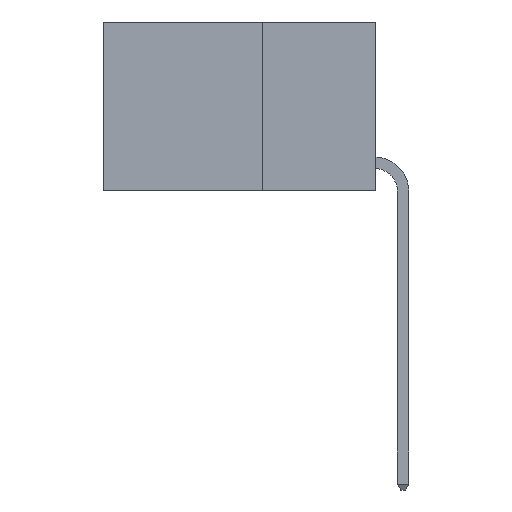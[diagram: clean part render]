
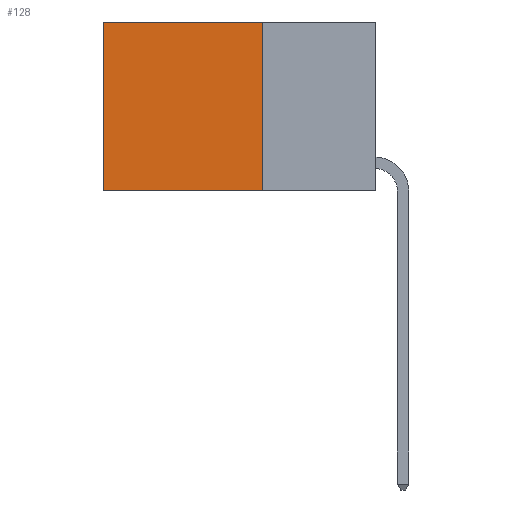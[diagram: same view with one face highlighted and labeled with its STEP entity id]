
A CAD part, left-side view. The second image highlights one B-rep face of the part: STEP entity #128.
In plain terms, the highlighted planar face has unit normal (-1, 0, 0).
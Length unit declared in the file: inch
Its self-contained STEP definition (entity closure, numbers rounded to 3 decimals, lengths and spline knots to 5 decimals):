
#128 = ADVANCED_FACE ( 'NONE', ( #4496 ), #8758, .F. ) ;
#533 = VECTOR ( 'NONE', #5621, 39.37008 ) ;
#545 = LINE ( 'NONE', #5864, #533 ) ;
#628 = EDGE_CURVE ( 'NONE', #7400, #764, #545, .T. ) ;
#734 = EDGE_LOOP ( 'NONE', ( #4826, #4939, #4992, #5083 ) ) ;
#764 = VERTEX_POINT ( 'NONE', #3080 ) ;
#966 = CARTESIAN_POINT ( 'NONE',  ( 0.2625, 0.25, 0. ) ) ;
#2362 = AXIS2_PLACEMENT_3D ( 'NONE', #4500, #7505, #8538 ) ;
#2675 = EDGE_CURVE ( 'NONE', #7400, #4387, #6437, .T. ) ;
#3080 = CARTESIAN_POINT ( 'NONE',  ( 0.2625, 0.25, -0.37 ) ) ;
#3181 = DIRECTION ( 'NONE',  ( 0., 1., 0. ) ) ;
#3272 = CARTESIAN_POINT ( 'NONE',  ( 0.2625, 0.25, 0. ) ) ;
#3732 = CARTESIAN_POINT ( 'NONE',  ( 0.2625, 0.6, -0.37 ) ) ;
#4236 = EDGE_CURVE ( 'NONE', #764, #8080, #7479, .T. ) ;
#4387 = VERTEX_POINT ( 'NONE', #5658 ) ;
#4496 = FACE_OUTER_BOUND ( 'NONE', #734, .T. ) ;
#4500 = CARTESIAN_POINT ( 'NONE',  ( 0.2625, 0.25, 0. ) ) ;
#4826 = ORIENTED_EDGE ( 'NONE', *, *, #4928, .T. ) ;
#4928 = EDGE_CURVE ( 'NONE', #4387, #8080, #5277, .T. ) ;
#4939 = ORIENTED_EDGE ( 'NONE', *, *, #4236, .F. ) ;
#4992 = ORIENTED_EDGE ( 'NONE', *, *, #628, .F. ) ;
#5083 = ORIENTED_EDGE ( 'NONE', *, *, #2675, .T. ) ;
#5277 = LINE ( 'NONE', #9057, #5325 ) ;
#5325 = VECTOR ( 'NONE', #9067, 39.37008 ) ;
#5621 = DIRECTION ( 'NONE',  ( 0., 0., -1. ) ) ;
#5658 = CARTESIAN_POINT ( 'NONE',  ( 0.2625, 0.6, 0. ) ) ;
#5864 = CARTESIAN_POINT ( 'NONE',  ( 0.2625, 0.25, 0. ) ) ;
#6437 = LINE ( 'NONE', #3272, #8177 ) ;
#7211 = VECTOR ( 'NONE', #8642, 39.37008 ) ;
#7400 = VERTEX_POINT ( 'NONE', #966 ) ;
#7479 = LINE ( 'NONE', #8477, #7211 ) ;
#7505 = DIRECTION ( 'NONE',  ( 1., 0., 0. ) ) ;
#8080 = VERTEX_POINT ( 'NONE', #3732 ) ;
#8177 = VECTOR ( 'NONE', #3181, 39.37008 ) ;
#8477 = CARTESIAN_POINT ( 'NONE',  ( 0.2625, 0.25, -0.37 ) ) ;
#8538 = DIRECTION ( 'NONE',  ( 0., 0., -1. ) ) ;
#8642 = DIRECTION ( 'NONE',  ( 0., 1., 0. ) ) ;
#8758 = PLANE ( 'NONE',  #2362 ) ;
#9057 = CARTESIAN_POINT ( 'NONE',  ( 0.2625, 0.6, 0. ) ) ;
#9067 = DIRECTION ( 'NONE',  ( 0., 0., -1. ) ) ;
